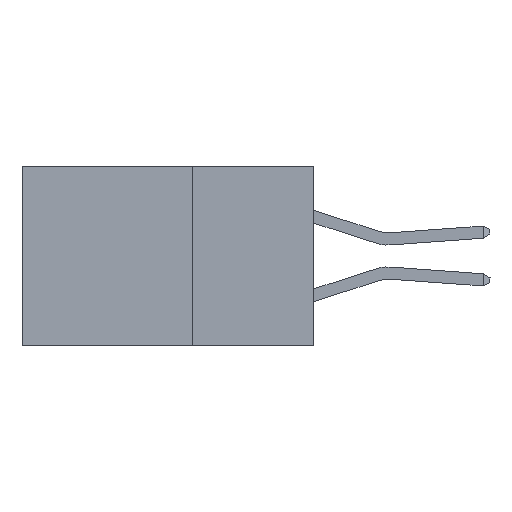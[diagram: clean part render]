
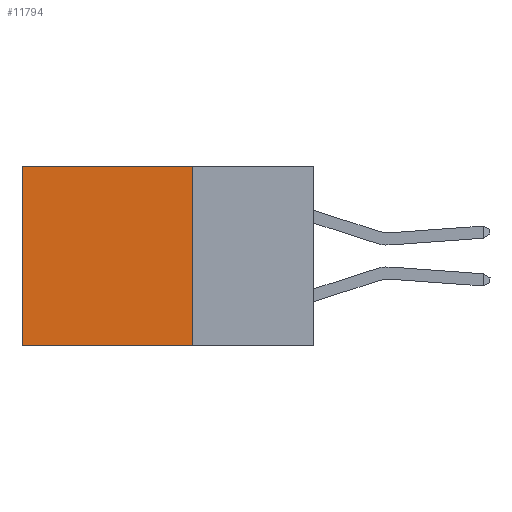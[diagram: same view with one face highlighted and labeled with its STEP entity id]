
A CAD part, left-side view. The second image highlights one B-rep face of the part: STEP entity #11794.
In plain terms, the highlighted planar face has unit normal (-1, 0, 0).
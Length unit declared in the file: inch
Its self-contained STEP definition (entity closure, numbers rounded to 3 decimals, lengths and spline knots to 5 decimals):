
#702 = ORIENTED_EDGE ( 'NONE', *, *, #16085, .T. ) ;
#1186 = VERTEX_POINT ( 'NONE', #13106 ) ;
#1319 = DIRECTION ( 'NONE',  ( 0., 1., 0. ) ) ;
#2397 = CARTESIAN_POINT ( 'NONE',  ( 0.2875, 0.6, -0.37 ) ) ;
#2431 = CARTESIAN_POINT ( 'NONE',  ( 0.2875, 0.6, 0. ) ) ;
#2447 = EDGE_LOOP ( 'NONE', ( #6211, #17291, #22828, #702 ) ) ;
#2497 = LINE ( 'NONE', #25716, #26831 ) ;
#6211 = ORIENTED_EDGE ( 'NONE', *, *, #23951, .T. ) ;
#7383 = VECTOR ( 'NONE', #1319, 39.37008 ) ;
#7851 = LINE ( 'NONE', #16162, #7383 ) ;
#8448 = VERTEX_POINT ( 'NONE', #2431 ) ;
#8933 = VERTEX_POINT ( 'NONE', #2397 ) ;
#9162 = FACE_OUTER_BOUND ( 'NONE', #2447, .T. ) ;
#11794 = ADVANCED_FACE ( 'NONE', ( #9162 ), #25614, .F. ) ;
#12299 = CARTESIAN_POINT ( 'NONE',  ( 0.2875, 0.25, -0.37 ) ) ;
#13087 = DIRECTION ( 'NONE',  ( 0., 0., -1. ) ) ;
#13106 = CARTESIAN_POINT ( 'NONE',  ( 0.2875, 0.25, 0. ) ) ;
#14861 = CARTESIAN_POINT ( 'NONE',  ( 0.2875, 0.25, 0. ) ) ;
#16085 = EDGE_CURVE ( 'NONE', #1186, #8448, #7851, .T. ) ;
#16162 = CARTESIAN_POINT ( 'NONE',  ( 0.2875, 0.25, 0. ) ) ;
#16674 = LINE ( 'NONE', #12299, #26004 ) ;
#16718 = VECTOR ( 'NONE', #23220, 39.37008 ) ;
#17011 = CARTESIAN_POINT ( 'NONE',  ( 0.2875, 0.25, -0.37 ) ) ;
#17249 = CARTESIAN_POINT ( 'NONE',  ( 0.2875, 0.25, 0. ) ) ;
#17291 = ORIENTED_EDGE ( 'NONE', *, *, #25064, .F. ) ;
#17520 = DIRECTION ( 'NONE',  ( 1., 0., 0. ) ) ;
#20759 = LINE ( 'NONE', #14861, #16718 ) ;
#22103 = AXIS2_PLACEMENT_3D ( 'NONE', #17249, #17520, #23558 ) ;
#22414 = EDGE_CURVE ( 'NONE', #1186, #26775, #20759, .T. ) ;
#22828 = ORIENTED_EDGE ( 'NONE', *, *, #22414, .F. ) ;
#23220 = DIRECTION ( 'NONE',  ( 0., 0., -1. ) ) ;
#23558 = DIRECTION ( 'NONE',  ( 0., 0., -1. ) ) ;
#23951 = EDGE_CURVE ( 'NONE', #8448, #8933, #2497, .T. ) ;
#25064 = EDGE_CURVE ( 'NONE', #26775, #8933, #16674, .T. ) ;
#25182 = DIRECTION ( 'NONE',  ( 0., 1., 0. ) ) ;
#25614 = PLANE ( 'NONE',  #22103 ) ;
#25716 = CARTESIAN_POINT ( 'NONE',  ( 0.2875, 0.6, 0. ) ) ;
#26004 = VECTOR ( 'NONE', #25182, 39.37008 ) ;
#26775 = VERTEX_POINT ( 'NONE', #17011 ) ;
#26831 = VECTOR ( 'NONE', #13087, 39.37008 ) ;
